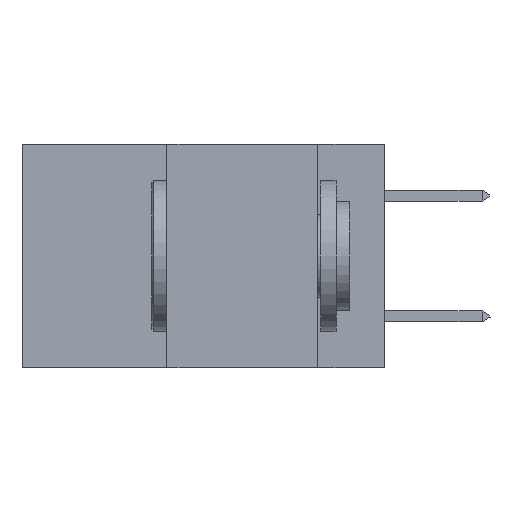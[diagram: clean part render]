
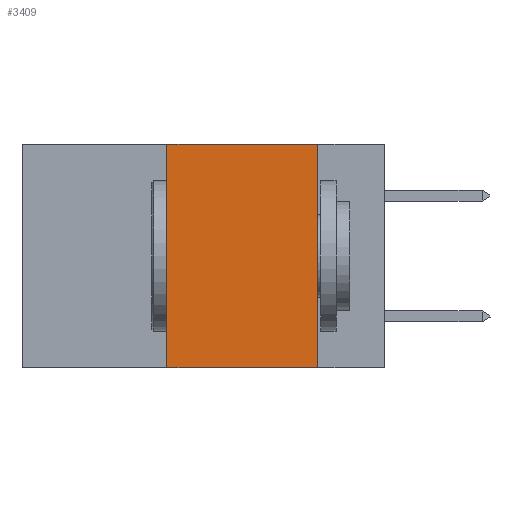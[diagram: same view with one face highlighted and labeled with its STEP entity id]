
A CAD part, left-side view. The second image highlights one B-rep face of the part: STEP entity #3409.
In plain terms, the highlighted planar face has unit normal (-1, 0, 0).
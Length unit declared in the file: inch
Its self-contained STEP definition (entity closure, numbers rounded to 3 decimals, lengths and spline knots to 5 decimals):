
#630 = ORIENTED_EDGE ( 'NONE', *, *, #2915, .T. ) ;
#1088 = VERTEX_POINT ( 'NONE', #4438 ) ;
#1289 = VECTOR ( 'NONE', #34884, 39.37008 ) ;
#2069 = CARTESIAN_POINT ( 'NONE',  ( 0., 0.36, -0.37 ) ) ;
#2754 = EDGE_CURVE ( 'NONE', #20216, #1088, #34495, .T. ) ;
#2915 = EDGE_CURVE ( 'NONE', #14817, #1088, #18867, .T. ) ;
#3244 = ORIENTED_EDGE ( 'NONE', *, *, #16175, .F. ) ;
#3409 = ADVANCED_FACE ( 'NONE', ( #25700 ), #9542, .F. ) ;
#4438 = CARTESIAN_POINT ( 'NONE',  ( 0., 0.11, -0.37 ) ) ;
#6819 = CARTESIAN_POINT ( 'NONE',  ( 0., 0.6, 0. ) ) ;
#7034 = CARTESIAN_POINT ( 'NONE',  ( 0., 0.6, -0.37 ) ) ;
#9542 = PLANE ( 'NONE',  #34980 ) ;
#9594 = VECTOR ( 'NONE', #22641, 39.37008 ) ;
#9928 = DIRECTION ( 'NONE',  ( 0., 0., -1. ) ) ;
#11267 = CARTESIAN_POINT ( 'NONE',  ( 0., 0.11, 0. ) ) ;
#12188 = DIRECTION ( 'NONE',  ( 0., 0., -1. ) ) ;
#13085 = DIRECTION ( 'NONE',  ( 1., 0., 0. ) ) ;
#13319 = CARTESIAN_POINT ( 'NONE',  ( 0., 0.36, 0. ) ) ;
#14817 = VERTEX_POINT ( 'NONE', #2069 ) ;
#16175 = EDGE_CURVE ( 'NONE', #22600, #20216, #27301, .T. ) ;
#16327 = EDGE_LOOP ( 'NONE', ( #16484, #3244, #36723, #630 ) ) ;
#16484 = ORIENTED_EDGE ( 'NONE', *, *, #2754, .F. ) ;
#18867 = LINE ( 'NONE', #7034, #1289 ) ;
#20216 = VERTEX_POINT ( 'NONE', #11267 ) ;
#22600 = VERTEX_POINT ( 'NONE', #23921 ) ;
#22641 = DIRECTION ( 'NONE',  ( 0., 0., 1. ) ) ;
#23921 = CARTESIAN_POINT ( 'NONE',  ( 0., 0.36, 0. ) ) ;
#24274 = VECTOR ( 'NONE', #12188, 39.37008 ) ;
#25700 = FACE_OUTER_BOUND ( 'NONE', #16327, .T. ) ;
#25894 = EDGE_CURVE ( 'NONE', #14817, #22600, #37902, .T. ) ;
#27301 = LINE ( 'NONE', #38567, #28269 ) ;
#28269 = VECTOR ( 'NONE', #32480, 39.37008 ) ;
#32480 = DIRECTION ( 'NONE',  ( 0., -1., 0. ) ) ;
#34495 = LINE ( 'NONE', #35974, #24274 ) ;
#34884 = DIRECTION ( 'NONE',  ( 0., -1., 0. ) ) ;
#34980 = AXIS2_PLACEMENT_3D ( 'NONE', #6819, #13085, #9928 ) ;
#35974 = CARTESIAN_POINT ( 'NONE',  ( 0., 0.11, 0. ) ) ;
#36723 = ORIENTED_EDGE ( 'NONE', *, *, #25894, .F. ) ;
#37902 = LINE ( 'NONE', #13319, #9594 ) ;
#38567 = CARTESIAN_POINT ( 'NONE',  ( 0., 0.6, 0. ) ) ;
